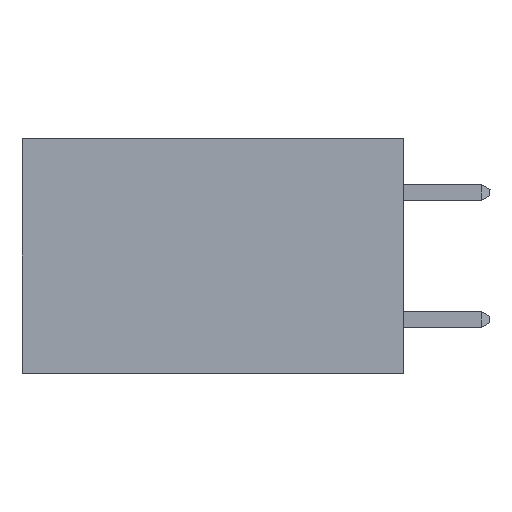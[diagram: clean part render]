
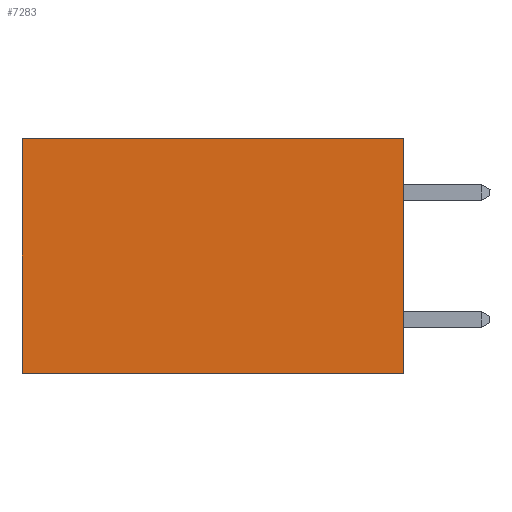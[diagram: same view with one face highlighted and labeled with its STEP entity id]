
A CAD part, left-side view. The second image highlights one B-rep face of the part: STEP entity #7283.
In plain terms, the highlighted planar face has unit normal (-1, 0, 0).
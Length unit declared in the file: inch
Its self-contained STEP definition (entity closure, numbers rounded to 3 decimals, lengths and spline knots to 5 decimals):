
#362 = PLANE ( 'NONE',  #16590 ) ;
#574 = DIRECTION ( 'NONE',  ( 0., 0., -1. ) ) ;
#1090 = VERTEX_POINT ( 'NONE', #13840 ) ;
#1753 = DIRECTION ( 'NONE',  ( 0., 0., -1. ) ) ;
#2278 = FACE_OUTER_BOUND ( 'NONE', #10765, .T. ) ;
#2378 = VECTOR ( 'NONE', #574, 39.37008 ) ;
#3704 = DIRECTION ( 'NONE',  ( 0., 1., 0. ) ) ;
#3940 = EDGE_CURVE ( 'NONE', #13054, #1090, #11904, .T. ) ;
#4165 = VECTOR ( 'NONE', #3704, 39.37008 ) ;
#5415 = VERTEX_POINT ( 'NONE', #15599 ) ;
#7283 = ADVANCED_FACE ( 'NONE', ( #2278 ), #362, .F. ) ;
#7341 = ORIENTED_EDGE ( 'NONE', *, *, #16313, .T. ) ;
#7459 = CARTESIAN_POINT ( 'NONE',  ( 0.2875, 0.6, 0. ) ) ;
#7571 = VECTOR ( 'NONE', #13450, 39.37008 ) ;
#7632 = CARTESIAN_POINT ( 'NONE',  ( 0.2875, 0., -0.37 ) ) ;
#8020 = CARTESIAN_POINT ( 'NONE',  ( 0.2875, 0., 0. ) ) ;
#8162 = EDGE_CURVE ( 'NONE', #5415, #1090, #16407, .T. ) ;
#9049 = LINE ( 'NONE', #8020, #7571 ) ;
#9259 = ORIENTED_EDGE ( 'NONE', *, *, #8162, .F. ) ;
#9290 = CARTESIAN_POINT ( 'NONE',  ( 0.2875, 0., 0. ) ) ;
#9426 = VERTEX_POINT ( 'NONE', #9290 ) ;
#9734 = ORIENTED_EDGE ( 'NONE', *, *, #3940, .T. ) ;
#10060 = DIRECTION ( 'NONE',  ( 1., 0., 0. ) ) ;
#10598 = ORIENTED_EDGE ( 'NONE', *, *, #11695, .F. ) ;
#10765 = EDGE_LOOP ( 'NONE', ( #9734, #9259, #10598, #7341 ) ) ;
#10831 = VECTOR ( 'NONE', #12555, 39.37008 ) ;
#11695 = EDGE_CURVE ( 'NONE', #9426, #5415, #9049, .T. ) ;
#11904 = LINE ( 'NONE', #7459, #2378 ) ;
#12555 = DIRECTION ( 'NONE',  ( 0., 1., 0. ) ) ;
#13054 = VERTEX_POINT ( 'NONE', #13881 ) ;
#13450 = DIRECTION ( 'NONE',  ( 0., 0., -1. ) ) ;
#13840 = CARTESIAN_POINT ( 'NONE',  ( 0.2875, 0.6, -0.37 ) ) ;
#13881 = CARTESIAN_POINT ( 'NONE',  ( 0.2875, 0.6, 0. ) ) ;
#15599 = CARTESIAN_POINT ( 'NONE',  ( 0.2875, 0., -0.37 ) ) ;
#16313 = EDGE_CURVE ( 'NONE', #9426, #13054, #16948, .T. ) ;
#16407 = LINE ( 'NONE', #7632, #4165 ) ;
#16487 = CARTESIAN_POINT ( 'NONE',  ( 0.2875, 0., 0. ) ) ;
#16590 = AXIS2_PLACEMENT_3D ( 'NONE', #16849, #10060, #1753 ) ;
#16849 = CARTESIAN_POINT ( 'NONE',  ( 0.2875, 0., 0. ) ) ;
#16948 = LINE ( 'NONE', #16487, #10831 ) ;
